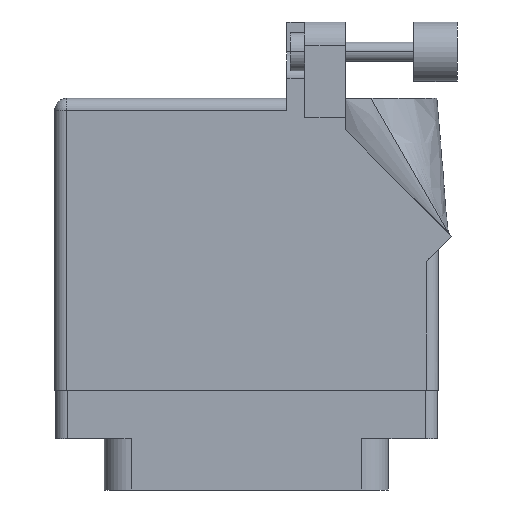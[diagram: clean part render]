
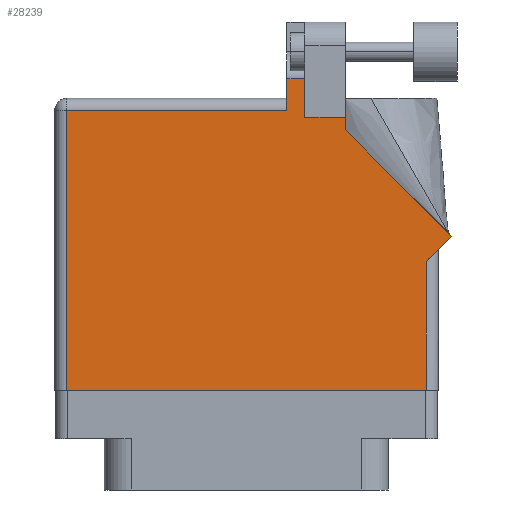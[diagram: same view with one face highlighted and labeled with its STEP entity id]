
A CAD part, front view. The second image highlights one B-rep face of the part: STEP entity #28239.
In plain terms, the highlighted face is planar.
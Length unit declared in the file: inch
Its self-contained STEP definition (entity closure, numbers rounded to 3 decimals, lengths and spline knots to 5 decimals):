
#36 = FACE_OUTER_BOUND ( 'NONE', #33407, .T. ) ;
#208 = VERTEX_POINT ( 'NONE', #40483 ) ;
#223 = VERTEX_POINT ( 'NONE', #9535 ) ;
#1543 = VERTEX_POINT ( 'NONE', #36097 ) ;
#1721 = EDGE_CURVE ( 'NONE', #13754, #34199, #1797, .T. ) ;
#1797 = LINE ( 'NONE', #2794, #34101 ) ;
#1899 = LINE ( 'NONE', #23986, #5815 ) ;
#2003 = DIRECTION ( 'NONE',  ( -1., 0., 0. ) ) ;
#2696 = DIRECTION ( 'NONE',  ( 0., -1., 0. ) ) ;
#2742 = EDGE_CURVE ( 'NONE', #34199, #8544, #1899, .T. ) ;
#2794 = CARTESIAN_POINT ( 'NONE',  ( -0.943, -0.1, 0.455 ) ) ;
#3903 = VECTOR ( 'NONE', #4191, 39.37008 ) ;
#4030 = ORIENTED_EDGE ( 'NONE', *, *, #21027, .T. ) ;
#4191 = DIRECTION ( 'NONE',  ( -1., 0., 0. ) ) ;
#5561 = LINE ( 'NONE', #14465, #27154 ) ;
#5815 = VECTOR ( 'NONE', #11480, 39.37008 ) ;
#5949 = EDGE_CURVE ( 'NONE', #208, #13754, #5561, .T. ) ;
#6101 = ORIENTED_EDGE ( 'NONE', *, *, #2742, .T. ) ;
#6187 = LINE ( 'NONE', #34742, #21891 ) ;
#6495 = CARTESIAN_POINT ( 'NONE',  ( -1.005, 1.43, 0.455 ) ) ;
#7565 = VERTEX_POINT ( 'NONE', #36331 ) ;
#8060 = DIRECTION ( 'NONE',  ( 0., 1., 0. ) ) ;
#8328 = LINE ( 'NONE', #38514, #10292 ) ;
#8544 = VERTEX_POINT ( 'NONE', #35675 ) ;
#8969 = CARTESIAN_POINT ( 'NONE',  ( 1.005, 0.637, 0.455 ) ) ;
#9535 = CARTESIAN_POINT ( 'NONE',  ( 0.212, 1.5315, 0.455 ) ) ;
#9767 = PLANE ( 'NONE',  #15262 ) ;
#10292 = VECTOR ( 'NONE', #23340, 39.37008 ) ;
#11480 = DIRECTION ( 'NONE',  ( 1., 0., 0. ) ) ;
#12746 = VECTOR ( 'NONE', #14608, 39.37008 ) ;
#13754 = VERTEX_POINT ( 'NONE', #39544 ) ;
#14109 = CARTESIAN_POINT ( 'NONE',  ( 0.943, 0.637, 0.455 ) ) ;
#14465 = CARTESIAN_POINT ( 'NONE',  ( -1.005, 1.368, 0.455 ) ) ;
#14608 = DIRECTION ( 'NONE',  ( -1., 0., 0. ) ) ;
#14677 = VECTOR ( 'NONE', #2696, 39.37008 ) ;
#14726 = LINE ( 'NONE', #27374, #12746 ) ;
#14917 = VERTEX_POINT ( 'NONE', #15266 ) ;
#15262 = AXIS2_PLACEMENT_3D ( 'NONE', #6495, #38278, #19504 ) ;
#15266 = CARTESIAN_POINT ( 'NONE',  ( 0.519, 1.33, 0.455 ) ) ;
#15468 = DIRECTION ( 'NONE',  ( -0.707, 0.707, 0. ) ) ;
#15538 = DIRECTION ( 'NONE',  ( 0., 1., 0. ) ) ;
#16762 = CARTESIAN_POINT ( 'NONE',  ( 0.943, 0.575, 0.455 ) ) ;
#17760 = CARTESIAN_POINT ( 'NONE',  ( 0.519, 1.26442, 0.455 ) ) ;
#19504 = DIRECTION ( 'NONE',  ( -1., 0., 0. ) ) ;
#20696 = ORIENTED_EDGE ( 'NONE', *, *, #5949, .T. ) ;
#21027 = EDGE_CURVE ( 'NONE', #7565, #223, #14726, .T. ) ;
#21891 = VECTOR ( 'NONE', #15468, 39.37008 ) ;
#22296 = VERTEX_POINT ( 'NONE', #17760 ) ;
#23340 = DIRECTION ( 'NONE',  ( 0., 1., 0. ) ) ;
#23824 = VECTOR ( 'NONE', #24787, 39.37008 ) ;
#23946 = ORIENTED_EDGE ( 'NONE', *, *, #32090, .T. ) ;
#23986 = CARTESIAN_POINT ( 'NONE',  ( -1.005, -0.1, 0.455 ) ) ;
#24787 = DIRECTION ( 'NONE',  ( 0.707, 0.707, 0. ) ) ;
#25449 = CARTESIAN_POINT ( 'NONE',  ( 0.306, 1.33, 0.455 ) ) ;
#26172 = ORIENTED_EDGE ( 'NONE', *, *, #30184, .T. ) ;
#26467 = ORIENTED_EDGE ( 'NONE', *, *, #37265, .T. ) ;
#26683 = ORIENTED_EDGE ( 'NONE', *, *, #36496, .T. ) ;
#26949 = VECTOR ( 'NONE', #8060, 39.37008 ) ;
#27154 = VECTOR ( 'NONE', #2003, 39.37008 ) ;
#27374 = CARTESIAN_POINT ( 'NONE',  ( 0.63677, 1.5315, 0.455 ) ) ;
#27735 = EDGE_CURVE ( 'NONE', #14917, #33427, #33812, .T. ) ;
#28032 = CARTESIAN_POINT ( 'NONE',  ( 0.212, 1.43, 0.455 ) ) ;
#28239 = ADVANCED_FACE ( 'NONE', ( #36 ), #9767, .F. ) ;
#28386 = CARTESIAN_POINT ( 'NONE',  ( 0.306, 1.33, 0.455 ) ) ;
#28974 = CARTESIAN_POINT ( 'NONE',  ( -0.943, -0.1, 0.455 ) ) ;
#29013 = ORIENTED_EDGE ( 'NONE', *, *, #32574, .T. ) ;
#29375 = LINE ( 'NONE', #14109, #26949 ) ;
#30184 = EDGE_CURVE ( 'NONE', #223, #208, #39658, .T. ) ;
#31218 = ORIENTED_EDGE ( 'NONE', *, *, #27735, .T. ) ;
#31321 = LINE ( 'NONE', #25449, #34289 ) ;
#31677 = VERTEX_POINT ( 'NONE', #16762 ) ;
#32090 = EDGE_CURVE ( 'NONE', #1543, #22296, #6187, .T. ) ;
#32410 = ORIENTED_EDGE ( 'NONE', *, *, #38083, .T. ) ;
#32574 = EDGE_CURVE ( 'NONE', #31677, #1543, #38969, .T. ) ;
#33407 = EDGE_LOOP ( 'NONE', ( #32410, #4030, #26172, #20696, #37242, #6101, #26467, #29013, #23946, #26683, #31218 ) ) ;
#33427 = VERTEX_POINT ( 'NONE', #28386 ) ;
#33812 = LINE ( 'NONE', #38469, #3903 ) ;
#34101 = VECTOR ( 'NONE', #37173, 39.37008 ) ;
#34199 = VERTEX_POINT ( 'NONE', #28974 ) ;
#34289 = VECTOR ( 'NONE', #15538, 39.37008 ) ;
#34742 = CARTESIAN_POINT ( 'NONE',  ( 1.07571, 0.70771, 0.455 ) ) ;
#35675 = CARTESIAN_POINT ( 'NONE',  ( 0.943, -0.1, 0.455 ) ) ;
#36097 = CARTESIAN_POINT ( 'NONE',  ( 1.07571, 0.70771, 0.455 ) ) ;
#36331 = CARTESIAN_POINT ( 'NONE',  ( 0.306, 1.5315, 0.455 ) ) ;
#36496 = EDGE_CURVE ( 'NONE', #22296, #14917, #8328, .T. ) ;
#37173 = DIRECTION ( 'NONE',  ( 0., -1., 0. ) ) ;
#37242 = ORIENTED_EDGE ( 'NONE', *, *, #1721, .T. ) ;
#37265 = EDGE_CURVE ( 'NONE', #8544, #31677, #29375, .T. ) ;
#38083 = EDGE_CURVE ( 'NONE', #33427, #7565, #31321, .T. ) ;
#38278 = DIRECTION ( 'NONE',  ( 0., 0., -1. ) ) ;
#38469 = CARTESIAN_POINT ( 'NONE',  ( 0.519, 1.33, 0.455 ) ) ;
#38514 = CARTESIAN_POINT ( 'NONE',  ( 0.519, 1.26442, 0.455 ) ) ;
#38969 = LINE ( 'NONE', #8969, #23824 ) ;
#39544 = CARTESIAN_POINT ( 'NONE',  ( -0.943, 1.368, 0.455 ) ) ;
#39658 = LINE ( 'NONE', #28032, #14677 ) ;
#40483 = CARTESIAN_POINT ( 'NONE',  ( 0.212, 1.368, 0.455 ) ) ;
